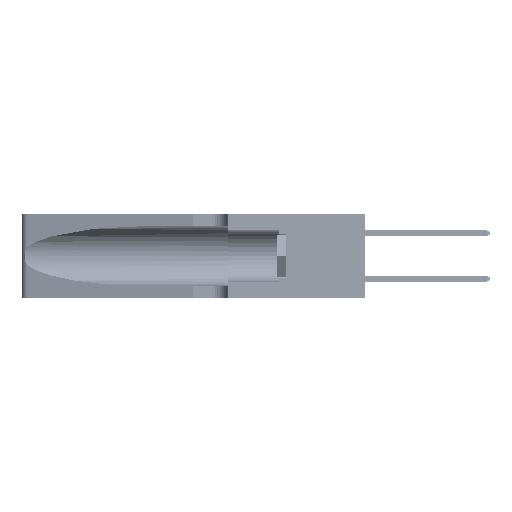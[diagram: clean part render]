
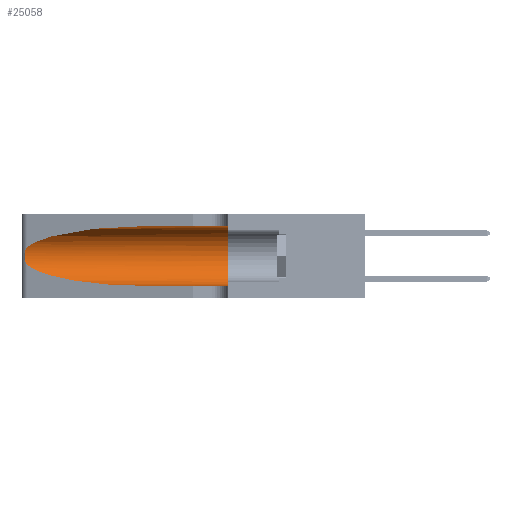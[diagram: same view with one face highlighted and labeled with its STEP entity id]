
A CAD part, left-side view. The second image highlights one B-rep face of the part: STEP entity #25058.
In plain terms, the highlighted cylindrical face has radius 3.308 mm (diameter 6.617 mm), a partial arc.
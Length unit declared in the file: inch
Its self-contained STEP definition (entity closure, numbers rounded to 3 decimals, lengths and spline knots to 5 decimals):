
#4526 = CARTESIAN_POINT ( 'NONE',  ( 0.26017, 1.23833, 0.17102 ) ) ;
#5235 = CYLINDRICAL_SURFACE ( 'NONE', #53672, 0.13025 ) ;
#5621 = CARTESIAN_POINT ( 'NONE',  ( 0.1305, 0.35, 0.31525 ) ) ;
#6135 = DIRECTION ( 'NONE',  ( 0., -1., 0. ) ) ;
#7161 = CARTESIAN_POINT ( 'NONE',  ( 0.25487, 1.22718, 0.14631 ) ) ;
#7465 = CARTESIAN_POINT ( 'NONE',  ( 0.1305, 0.35, 0.05475 ) ) ;
#7973 = CARTESIAN_POINT ( 'NONE',  ( 0.25856, 1.23593, 0.16098 ) ) ;
#11277 = EDGE_LOOP ( 'NONE', ( #36058, #45582, #18396, #23545, #39734, #34462 ) ) ;
#11664 = CARTESIAN_POINT ( 'NONE',  ( 0.25487, 1.22718, 0.14631 ) ) ;
#11992 = CARTESIAN_POINT ( 'NONE',  ( 0.25639, 1.23186, 0.15144 ) ) ;
#12213 = CARTESIAN_POINT ( 'NONE',  ( 0.1305, 1.61858, 0.185 ) ) ;
#15534 = LINE ( 'NONE', #38987, #40368 ) ;
#16044 = VERTEX_POINT ( 'NONE', #5621 ) ;
#16563 = DIRECTION ( 'NONE',  ( 0., -1., 0. ) ) ;
#16686 = CARTESIAN_POINT ( 'NONE',  ( 0.25639, 1.23184, 0.21858 ) ) ;
#16928 = CARTESIAN_POINT ( 'NONE',  ( 0.1305, 1.61858, 0.05475 ) ) ;
#18396 = ORIENTED_EDGE ( 'NONE', *, *, #41574, .T. ) ;
#19255 = EDGE_CURVE ( 'NONE', #34670, #16044, #15534, .T. ) ;
#20320 = CARTESIAN_POINT ( 'NONE',  ( 0.26075, 1.23896, 0.178 ) ) ;
#21616 = VERTEX_POINT ( 'NONE', #7465 ) ;
#22144 = VECTOR ( 'NONE', #25139, 39.37008 ) ;
#23545 = ORIENTED_EDGE ( 'NONE', *, *, #45791, .T. ) ;
#24364 = CARTESIAN_POINT ( 'NONE',  ( 0.1305, 0.72297, 0.31525 ) ) ;
#24948 = DIRECTION ( 'NONE',  ( 0., 0., -1. ) ) ;
#25058 = ADVANCED_FACE ( 'NONE', ( #31355 ), #5235, .F. ) ;
#25100 = CARTESIAN_POINT ( 'NONE',  ( 0.1305, 0.72297, 0.31525 ) ) ;
#25139 = DIRECTION ( 'NONE',  ( 0., -1., 0. ) ) ;
#25259 = DIRECTION ( 'NONE',  ( 0., 0., 1. ) ) ;
#25424 = AXIS2_PLACEMENT_3D ( 'NONE', #29302, #45509, #25259 ) ;
#27555 = VERTEX_POINT ( 'NONE', #7161 ) ;
#28957 = CARTESIAN_POINT ( 'NONE',  ( 0.25555, 1.22993, 0.14849 ) ) ;
#29302 = CARTESIAN_POINT ( 'NONE',  ( 0.1305, 0.35, 0.185 ) ) ;
#29480 = CARTESIAN_POINT ( 'NONE',  ( 0.25487, 1.22718, 0.14631 ) ) ;
#29541 = VERTEX_POINT ( 'NONE', #42639 ) ;
#31355 = FACE_OUTER_BOUND ( 'NONE', #11277, .T. ) ;
#32015 =( BOUNDED_CURVE ( )  B_SPLINE_CURVE ( 3, ( #24364, #53773, #42271, #53951 ),
 .UNSPECIFIED., .F., .T. ) 
 B_SPLINE_CURVE_WITH_KNOTS ( ( 4, 4 ),
 ( 1.5708, 2.84003 ),
 .UNSPECIFIED. ) 
 CURVE ( )  GEOMETRIC_REPRESENTATION_ITEM ( )  RATIONAL_B_SPLINE_CURVE ( ( 1., 0.87, 0.87, 1. ) ) 
 REPRESENTATION_ITEM ( '' )  );
#32958 = CARTESIAN_POINT ( 'NONE',  ( 0.26018, 1.23835, 0.19895 ) ) ;
#33135 = CARTESIAN_POINT ( 'NONE',  ( 0.25487, 1.22718, 0.22369 ) ) ;
#34462 = ORIENTED_EDGE ( 'NONE', *, *, #19255, .F. ) ;
#34670 = VERTEX_POINT ( 'NONE', #25100 ) ;
#36058 = ORIENTED_EDGE ( 'NONE', *, *, #36130, .T. ) ;
#36130 = EDGE_CURVE ( 'NONE', #34670, #42578, #32015, .T. ) ;
#37360 = CARTESIAN_POINT ( 'NONE',  ( 0.26075, 1.23896, 0.19203 ) ) ;
#38987 = CARTESIAN_POINT ( 'NONE',  ( 0.1305, 1.61858, 0.31525 ) ) ;
#39734 = ORIENTED_EDGE ( 'NONE', *, *, #39892, .F. ) ;
#39892 = EDGE_CURVE ( 'NONE', #16044, #21616, #52197, .T. ) ;
#39967 = EDGE_CURVE ( 'NONE', #42578, #27555, #41665, .T. ) ;
#40309 = CARTESIAN_POINT ( 'NONE',  ( 0.1305, 0.72297, 0.05475 ) ) ;
#40368 = VECTOR ( 'NONE', #6135, 39.37008 ) ;
#41574 = EDGE_CURVE ( 'NONE', #27555, #29541, #49711, .T. ) ;
#41665 = B_SPLINE_CURVE_WITH_KNOTS ( 'NONE', 3,
 ( #33135, #46070, #16686, #53765, #50107, #32958, #37360, #20320, #4526, #7973, #50280, #11992, #28957, #29480 ),
 .UNSPECIFIED., .F., .F.,
 ( 4, 2, 2, 2, 2, 2, 4 ),
 ( 0., 0.00027, 0.00053, 0.00107, 0.0016, 0.00187, 0.00214 ),
 .UNSPECIFIED. ) ;
#42271 = CARTESIAN_POINT ( 'NONE',  ( 0.2373, 1.15595, 0.28018 ) ) ;
#42578 = VERTEX_POINT ( 'NONE', #45700 ) ;
#42639 = CARTESIAN_POINT ( 'NONE',  ( 0.1305, 0.72297, 0.05475 ) ) ;
#44369 = LINE ( 'NONE', #16928, #22144 ) ;
#45006 = CARTESIAN_POINT ( 'NONE',  ( 0.18966, 0.96281, 0.05475 ) ) ;
#45509 = DIRECTION ( 'NONE',  ( 0., 1., 0. ) ) ;
#45582 = ORIENTED_EDGE ( 'NONE', *, *, #39967, .T. ) ;
#45700 = CARTESIAN_POINT ( 'NONE',  ( 0.25487, 1.22718, 0.22369 ) ) ;
#45791 = EDGE_CURVE ( 'NONE', #29541, #21616, #44369, .T. ) ;
#46070 = CARTESIAN_POINT ( 'NONE',  ( 0.25555, 1.22994, 0.2215 ) ) ;
#48526 = CARTESIAN_POINT ( 'NONE',  ( 0.2373, 1.15595, 0.08982 ) ) ;
#49711 =( BOUNDED_CURVE ( )  B_SPLINE_CURVE ( 3, ( #11664, #48526, #45006, #40309 ),
 .UNSPECIFIED., .F., .F. ) 
 B_SPLINE_CURVE_WITH_KNOTS ( ( 4, 4 ),
 ( 3.44316, 4.71239 ),
 .UNSPECIFIED. ) 
 CURVE ( )  GEOMETRIC_REPRESENTATION_ITEM ( )  RATIONAL_B_SPLINE_CURVE ( ( 1., 0.87, 0.87, 1. ) ) 
 REPRESENTATION_ITEM ( '' )  );
#50107 = CARTESIAN_POINT ( 'NONE',  ( 0.25854, 1.2359, 0.20912 ) ) ;
#50280 = CARTESIAN_POINT ( 'NONE',  ( 0.25789, 1.23486, 0.15765 ) ) ;
#52197 = CIRCLE ( 'NONE', #25424, 0.13025 ) ;
#53672 = AXIS2_PLACEMENT_3D ( 'NONE', #12213, #16563, #24948 ) ;
#53765 = CARTESIAN_POINT ( 'NONE',  ( 0.25787, 1.23484, 0.2124 ) ) ;
#53773 = CARTESIAN_POINT ( 'NONE',  ( 0.18966, 0.96281, 0.31525 ) ) ;
#53951 = CARTESIAN_POINT ( 'NONE',  ( 0.25487, 1.22718, 0.22369 ) ) ;
